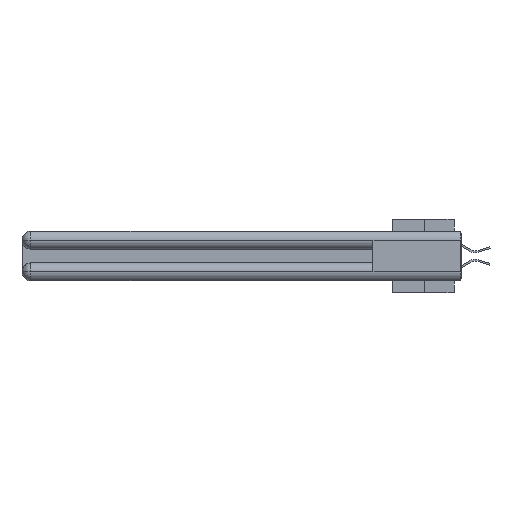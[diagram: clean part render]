
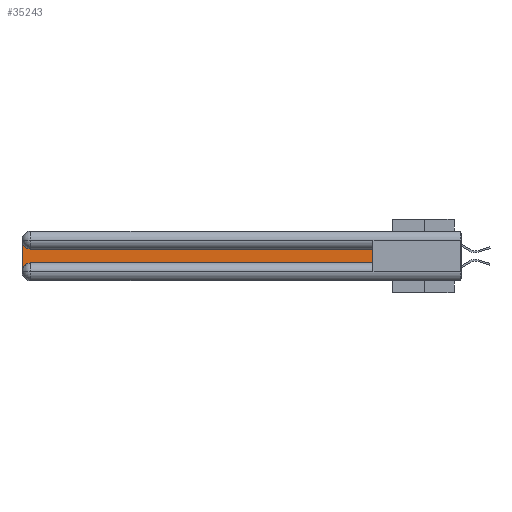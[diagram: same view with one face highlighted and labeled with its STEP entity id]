
A CAD part, left-side view. The second image highlights one B-rep face of the part: STEP entity #35243.
In plain terms, the highlighted planar face has unit normal (-1, 0, 0).
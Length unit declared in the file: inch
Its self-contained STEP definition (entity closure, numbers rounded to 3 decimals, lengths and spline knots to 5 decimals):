
#98 = CIRCLE ( 'NONE', #25323, 0.06 ) ;
#129 = ORIENTED_EDGE ( 'NONE', *, *, #9739, .T. ) ;
#256 = CARTESIAN_POINT ( 'NONE',  ( 0.075, 2.94, -0.2775 ) ) ;
#300 = DIRECTION ( 'NONE',  ( 0., 0., 1. ) ) ;
#559 = VERTEX_POINT ( 'NONE', #27814 ) ;
#807 = LINE ( 'NONE', #11768, #16815 ) ;
#834 = EDGE_CURVE ( 'NONE', #2626, #27089, #15749, .T. ) ;
#843 = CARTESIAN_POINT ( 'NONE',  ( 0.075, 0.6, -0.1225 ) ) ;
#1527 = CARTESIAN_POINT ( 'NONE',  ( 0.075, 3., -0.0625 ) ) ;
#1692 = CARTESIAN_POINT ( 'NONE',  ( 0.075, 2.94, -0.0625 ) ) ;
#2017 = FACE_OUTER_BOUND ( 'NONE', #31318, .T. ) ;
#2626 = VERTEX_POINT ( 'NONE', #843 ) ;
#2944 = DIRECTION ( 'NONE',  ( 1., 0., 0. ) ) ;
#4533 = DIRECTION ( 'NONE',  ( 1., 0., 0. ) ) ;
#4562 = EDGE_CURVE ( 'NONE', #6804, #559, #28043, .T. ) ;
#5429 = ORIENTED_EDGE ( 'NONE', *, *, #834, .T. ) ;
#6348 = ORIENTED_EDGE ( 'NONE', *, *, #7017, .T. ) ;
#6804 = VERTEX_POINT ( 'NONE', #22744 ) ;
#7017 = EDGE_CURVE ( 'NONE', #27089, #34732, #98, .T. ) ;
#7272 = DIRECTION ( 'NONE',  ( 0., 0., -1. ) ) ;
#7993 = EDGE_CURVE ( 'NONE', #559, #2626, #10547, .T. ) ;
#9739 = EDGE_CURVE ( 'NONE', #34732, #28277, #807, .T. ) ;
#10547 = LINE ( 'NONE', #27451, #31152 ) ;
#11458 = EDGE_CURVE ( 'NONE', #28277, #6804, #24934, .T. ) ;
#11768 = CARTESIAN_POINT ( 'NONE',  ( 0.075, 3., -0.2175 ) ) ;
#12671 = DIRECTION ( 'NONE',  ( 0., 1., 0. ) ) ;
#14205 = CARTESIAN_POINT ( 'NONE',  ( 0.075, 0.6, -0.2175 ) ) ;
#15749 = LINE ( 'NONE', #18265, #35302 ) ;
#16815 = VECTOR ( 'NONE', #31719, 39.37008 ) ;
#18265 = CARTESIAN_POINT ( 'NONE',  ( 0.075, 0.6, -0.1225 ) ) ;
#19203 = AXIS2_PLACEMENT_3D ( 'NONE', #256, #2944, #28272 ) ;
#20530 = PLANE ( 'NONE',  #32359 ) ;
#22744 = CARTESIAN_POINT ( 'NONE',  ( 0.075, 2.94, -0.2175 ) ) ;
#24276 = VECTOR ( 'NONE', #30923, 39.37008 ) ;
#24934 = CIRCLE ( 'NONE', #19203, 0.06 ) ;
#25287 = ORIENTED_EDGE ( 'NONE', *, *, #4562, .T. ) ;
#25323 = AXIS2_PLACEMENT_3D ( 'NONE', #1692, #31908, #7272 ) ;
#26008 = ORIENTED_EDGE ( 'NONE', *, *, #11458, .T. ) ;
#26099 = DIRECTION ( 'NONE',  ( 0., 0., -1. ) ) ;
#26637 = CARTESIAN_POINT ( 'NONE',  ( 0.075, 3., -0.1225 ) ) ;
#27089 = VERTEX_POINT ( 'NONE', #27341 ) ;
#27341 = CARTESIAN_POINT ( 'NONE',  ( 0.075, 2.94, -0.1225 ) ) ;
#27451 = CARTESIAN_POINT ( 'NONE',  ( 0.075, 0.6, -0.2175 ) ) ;
#27814 = CARTESIAN_POINT ( 'NONE',  ( 0.075, 0.6, -0.2175 ) ) ;
#28043 = LINE ( 'NONE', #14205, #24276 ) ;
#28272 = DIRECTION ( 'NONE',  ( 0., 0., -1. ) ) ;
#28277 = VERTEX_POINT ( 'NONE', #29144 ) ;
#29144 = CARTESIAN_POINT ( 'NONE',  ( 0.075, 3., -0.2775 ) ) ;
#30923 = DIRECTION ( 'NONE',  ( 0., -1., 0. ) ) ;
#31152 = VECTOR ( 'NONE', #300, 39.37008 ) ;
#31318 = EDGE_LOOP ( 'NONE', ( #5429, #6348, #129, #26008, #25287, #31950 ) ) ;
#31719 = DIRECTION ( 'NONE',  ( 0., 0., -1. ) ) ;
#31908 = DIRECTION ( 'NONE',  ( 1., 0., 0. ) ) ;
#31950 = ORIENTED_EDGE ( 'NONE', *, *, #7993, .T. ) ;
#32359 = AXIS2_PLACEMENT_3D ( 'NONE', #26637, #4533, #26099 ) ;
#34732 = VERTEX_POINT ( 'NONE', #1527 ) ;
#35243 = ADVANCED_FACE ( 'NONE', ( #2017 ), #20530, .F. ) ;
#35302 = VECTOR ( 'NONE', #12671, 39.37008 ) ;
